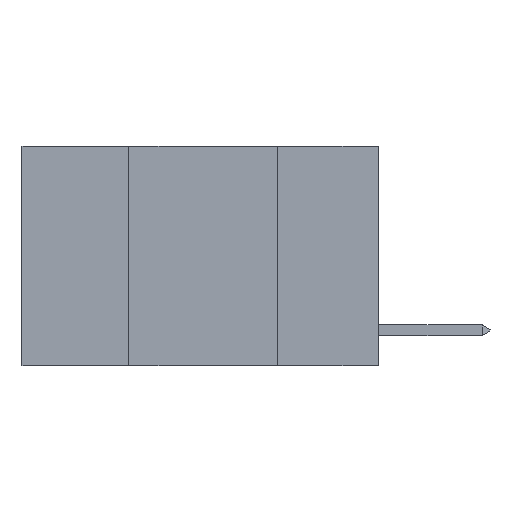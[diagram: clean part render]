
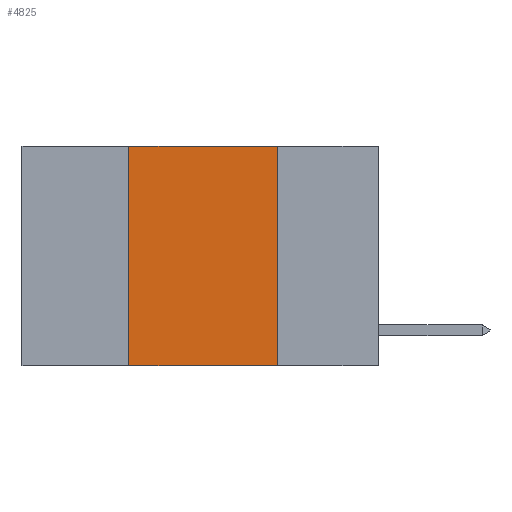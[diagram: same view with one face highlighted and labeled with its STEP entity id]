
A CAD part, left-side view. The second image highlights one B-rep face of the part: STEP entity #4825.
In plain terms, the highlighted planar face has unit normal (-1, 0, 0).
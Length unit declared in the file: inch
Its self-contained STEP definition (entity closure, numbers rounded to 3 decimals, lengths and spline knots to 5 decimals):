
#123 = LINE ( 'NONE', #9155, #20184 ) ;
#246 = ORIENTED_EDGE ( 'NONE', *, *, #16663, .F. ) ;
#790 = VECTOR ( 'NONE', #14259, 39.37008 ) ;
#805 = EDGE_CURVE ( 'NONE', #6338, #12467, #11634, .T. ) ;
#1003 = ORIENTED_EDGE ( 'NONE', *, *, #3520, .T. ) ;
#1394 = PLANE ( 'NONE',  #13205 ) ;
#2574 = EDGE_CURVE ( 'NONE', #12412, #11850, #17950, .T. ) ;
#2867 = ORIENTED_EDGE ( 'NONE', *, *, #2574, .F. ) ;
#2951 = ORIENTED_EDGE ( 'NONE', *, *, #805, .F. ) ;
#3022 = CARTESIAN_POINT ( 'NONE',  ( 0., 0.6, 0. ) ) ;
#3135 = CARTESIAN_POINT ( 'NONE',  ( 0., 0.6, -0.37 ) ) ;
#3520 = EDGE_CURVE ( 'NONE', #12412, #12467, #17677, .T. ) ;
#4649 = DIRECTION ( 'NONE',  ( 0., 0., -1. ) ) ;
#4825 = ADVANCED_FACE ( 'NONE', ( #17622 ), #1394, .F. ) ;
#4898 = EDGE_LOOP ( 'NONE', ( #2951, #246, #2867, #1003 ) ) ;
#6338 = VERTEX_POINT ( 'NONE', #7233 ) ;
#7233 = CARTESIAN_POINT ( 'NONE',  ( 0., 0.17, 0. ) ) ;
#8865 = CARTESIAN_POINT ( 'NONE',  ( 0., 0.42, 0. ) ) ;
#8979 = CARTESIAN_POINT ( 'NONE',  ( 0., 0.42, 0. ) ) ;
#9155 = CARTESIAN_POINT ( 'NONE',  ( 0., 0.6, 0. ) ) ;
#9157 = DIRECTION ( 'NONE',  ( 0., 0., 1. ) ) ;
#10146 = DIRECTION ( 'NONE',  ( 0., 0., -1. ) ) ;
#10651 = CARTESIAN_POINT ( 'NONE',  ( 0., 0.17, 0. ) ) ;
#10755 = DIRECTION ( 'NONE',  ( 0., -1., 0. ) ) ;
#11634 = LINE ( 'NONE', #10651, #19426 ) ;
#11850 = VERTEX_POINT ( 'NONE', #8865 ) ;
#12412 = VERTEX_POINT ( 'NONE', #14946 ) ;
#12467 = VERTEX_POINT ( 'NONE', #19716 ) ;
#13205 = AXIS2_PLACEMENT_3D ( 'NONE', #3022, #14156, #4649 ) ;
#13832 = VECTOR ( 'NONE', #9157, 39.37008 ) ;
#14156 = DIRECTION ( 'NONE',  ( 1., 0., 0. ) ) ;
#14259 = DIRECTION ( 'NONE',  ( 0., -1., 0. ) ) ;
#14946 = CARTESIAN_POINT ( 'NONE',  ( 0., 0.42, -0.37 ) ) ;
#16663 = EDGE_CURVE ( 'NONE', #11850, #6338, #123, .T. ) ;
#17622 = FACE_OUTER_BOUND ( 'NONE', #4898, .T. ) ;
#17677 = LINE ( 'NONE', #3135, #790 ) ;
#17950 = LINE ( 'NONE', #8979, #13832 ) ;
#19426 = VECTOR ( 'NONE', #10146, 39.37008 ) ;
#19716 = CARTESIAN_POINT ( 'NONE',  ( 0., 0.17, -0.37 ) ) ;
#20184 = VECTOR ( 'NONE', #10755, 39.37008 ) ;
